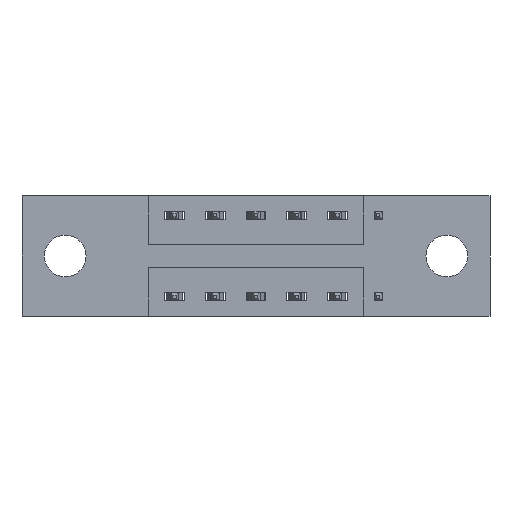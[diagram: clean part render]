
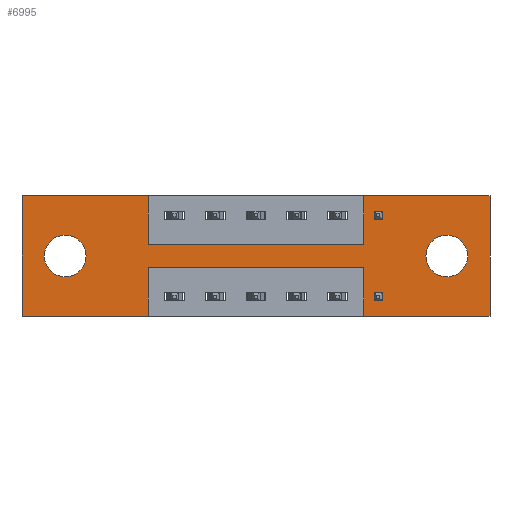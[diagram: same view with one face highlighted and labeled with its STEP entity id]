
A CAD part, front view. The second image highlights one B-rep face of the part: STEP entity #6995.
In plain terms, the highlighted planar face has unit normal (0, -1, 0).
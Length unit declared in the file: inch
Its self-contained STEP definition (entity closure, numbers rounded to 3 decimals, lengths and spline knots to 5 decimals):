
#26 = VERTEX_POINT ( 'NONE', #4920 ) ;
#130 = DIRECTION ( 'NONE',  ( 0., 0., -1. ) ) ;
#154 = CIRCLE ( 'NONE', #3363, 0.064 ) ;
#184 = AXIS2_PLACEMENT_3D ( 'NONE', #5138, #247, #5956 ) ;
#207 = ORIENTED_EDGE ( 'NONE', *, *, #250, .F. ) ;
#247 = DIRECTION ( 'NONE',  ( 0., -1., 0. ) ) ;
#250 = EDGE_CURVE ( 'NONE', #4261, #26, #7551, .T. ) ;
#269 = CARTESIAN_POINT ( 'NONE',  ( 0., 0., 0. ) ) ;
#484 = LINE ( 'NONE', #3034, #7723 ) ;
#500 = VERTEX_POINT ( 'NONE', #683 ) ;
#508 = EDGE_CURVE ( 'NONE', #796, #6614, #5262, .T. ) ;
#578 = AXIS2_PLACEMENT_3D ( 'NONE', #3106, #1083, #6284 ) ;
#643 = EDGE_CURVE ( 'NONE', #3928, #4161, #154, .T. ) ;
#683 = CARTESIAN_POINT ( 'NONE',  ( 0., 0., 0. ) ) ;
#751 = CARTESIAN_POINT ( 'NONE',  ( 1.3025, 0., -0.185 ) ) ;
#796 = VERTEX_POINT ( 'NONE', #7041 ) ;
#982 = ORIENTED_EDGE ( 'NONE', *, *, #6462, .F. ) ;
#998 = ORIENTED_EDGE ( 'NONE', *, *, #5204, .F. ) ;
#1083 = DIRECTION ( 'NONE',  ( 0., 1., 0. ) ) ;
#1354 = ORIENTED_EDGE ( 'NONE', *, *, #7322, .F. ) ;
#1363 = VERTEX_POINT ( 'NONE', #4975 ) ;
#1397 = DIRECTION ( 'NONE',  ( 0., 0., 1. ) ) ;
#1439 = CARTESIAN_POINT ( 'NONE',  ( 1.0475, 0., -0.15 ) ) ;
#1505 = DIRECTION ( 'NONE',  ( 0., 1., 0. ) ) ;
#1611 = ORIENTED_EDGE ( 'NONE', *, *, #8001, .F. ) ;
#1653 = VECTOR ( 'NONE', #5224, 39.37008 ) ;
#1746 = CARTESIAN_POINT ( 'NONE',  ( 1.435, 0., 0. ) ) ;
#1780 = VECTOR ( 'NONE', #1831, 39.37008 ) ;
#1831 = DIRECTION ( 'NONE',  ( 0., 0., 1. ) ) ;
#1835 = VERTEX_POINT ( 'NONE', #4892 ) ;
#1942 = CARTESIAN_POINT ( 'NONE',  ( 1.3025, 0., -0.249 ) ) ;
#2013 = LINE ( 'NONE', #3412, #4089 ) ;
#2039 = VECTOR ( 'NONE', #6839, 39.37008 ) ;
#2126 = LINE ( 'NONE', #2220, #7481 ) ;
#2173 = FACE_BOUND ( 'NONE', #6043, .T. ) ;
#2220 = CARTESIAN_POINT ( 'NONE',  ( 0., 0., -0.37 ) ) ;
#2291 = AXIS2_PLACEMENT_3D ( 'NONE', #4592, #7200, #1397 ) ;
#2400 = LINE ( 'NONE', #1746, #3653 ) ;
#2401 = DIRECTION ( 'NONE',  ( 1., 0., 0. ) ) ;
#2428 = CARTESIAN_POINT ( 'NONE',  ( 0., 0., 0. ) ) ;
#2572 = FACE_BOUND ( 'NONE', #6001, .T. ) ;
#2657 = CARTESIAN_POINT ( 'NONE',  ( 0.3875, 0., 0. ) ) ;
#2852 = DIRECTION ( 'NONE',  ( -1., 0., 0. ) ) ;
#3034 = CARTESIAN_POINT ( 'NONE',  ( 0.3875, 0., -0.37 ) ) ;
#3106 = CARTESIAN_POINT ( 'NONE',  ( 1.3025, 0., -0.185 ) ) ;
#3128 = ORIENTED_EDGE ( 'NONE', *, *, #6945, .F. ) ;
#3243 = EDGE_CURVE ( 'NONE', #6526, #500, #4103, .T. ) ;
#3318 = DIRECTION ( 'NONE',  ( 0., 1., 0. ) ) ;
#3351 = CARTESIAN_POINT ( 'NONE',  ( 0., 0., -0.37 ) ) ;
#3363 = AXIS2_PLACEMENT_3D ( 'NONE', #751, #3318, #130 ) ;
#3412 = CARTESIAN_POINT ( 'NONE',  ( 1.0475, 0., 0. ) ) ;
#3513 = EDGE_CURVE ( 'NONE', #5589, #1835, #5883, .T. ) ;
#3555 = CARTESIAN_POINT ( 'NONE',  ( 1.0475, 0., 0. ) ) ;
#3630 = LINE ( 'NONE', #4946, #5316 ) ;
#3653 = VECTOR ( 'NONE', #4329, 39.37008 ) ;
#3655 = ORIENTED_EDGE ( 'NONE', *, *, #508, .T. ) ;
#3745 = LINE ( 'NONE', #4406, #5836 ) ;
#3862 = ORIENTED_EDGE ( 'NONE', *, *, #6370, .F. ) ;
#3868 = LINE ( 'NONE', #6358, #1780 ) ;
#3928 = VERTEX_POINT ( 'NONE', #6560 ) ;
#4005 = DIRECTION ( 'NONE',  ( -1., 0., 0. ) ) ;
#4089 = VECTOR ( 'NONE', #4628, 39.37008 ) ;
#4103 = LINE ( 'NONE', #269, #5554 ) ;
#4123 = ORIENTED_EDGE ( 'NONE', *, *, #5888, .F. ) ;
#4161 = VERTEX_POINT ( 'NONE', #1942 ) ;
#4261 = VERTEX_POINT ( 'NONE', #3555 ) ;
#4328 = VECTOR ( 'NONE', #4005, 39.37008 ) ;
#4329 = DIRECTION ( 'NONE',  ( 0., 0., -1. ) ) ;
#4406 = CARTESIAN_POINT ( 'NONE',  ( 0., 0., 0. ) ) ;
#4583 = CARTESIAN_POINT ( 'NONE',  ( 0.3875, 0., -0.22 ) ) ;
#4592 = CARTESIAN_POINT ( 'NONE',  ( 0.1325, 0., -0.185 ) ) ;
#4628 = DIRECTION ( 'NONE',  ( 0., 0., 1. ) ) ;
#4744 = CARTESIAN_POINT ( 'NONE',  ( 0.3875, 0., -0.37 ) ) ;
#4803 = DIRECTION ( 'NONE',  ( 0., 0., 1. ) ) ;
#4891 = CARTESIAN_POINT ( 'NONE',  ( 0.3875, 0., -0.15 ) ) ;
#4892 = CARTESIAN_POINT ( 'NONE',  ( 0.3875, 0., -0.15 ) ) ;
#4894 = AXIS2_PLACEMENT_3D ( 'NONE', #7319, #1505, #6663 ) ;
#4920 = CARTESIAN_POINT ( 'NONE',  ( 1.435, 0., 0. ) ) ;
#4946 = CARTESIAN_POINT ( 'NONE',  ( 0., 0., -0.37 ) ) ;
#4975 = CARTESIAN_POINT ( 'NONE',  ( 1.0475, 0., -0.37 ) ) ;
#5138 = CARTESIAN_POINT ( 'NONE',  ( 0., 0., -0.37 ) ) ;
#5180 = EDGE_CURVE ( 'NONE', #4161, #3928, #6217, .T. ) ;
#5204 = EDGE_CURVE ( 'NONE', #26, #7951, #2400, .T. ) ;
#5205 = ORIENTED_EDGE ( 'NONE', *, *, #643, .T. ) ;
#5224 = DIRECTION ( 'NONE',  ( 0., 0., -1. ) ) ;
#5260 = ORIENTED_EDGE ( 'NONE', *, *, #5180, .T. ) ;
#5262 = CIRCLE ( 'NONE', #2291, 0.064 ) ;
#5316 = VECTOR ( 'NONE', #7529, 39.37008 ) ;
#5353 = PLANE ( 'NONE',  #184 ) ;
#5452 = CARTESIAN_POINT ( 'NONE',  ( 1.0475, 0., -0.22 ) ) ;
#5457 = ORIENTED_EDGE ( 'NONE', *, *, #8246, .F. ) ;
#5554 = VECTOR ( 'NONE', #4803, 39.37008 ) ;
#5589 = VERTEX_POINT ( 'NONE', #8318 ) ;
#5612 = DIRECTION ( 'NONE',  ( 0., 0., -1. ) ) ;
#5786 = FACE_OUTER_BOUND ( 'NONE', #6097, .T. ) ;
#5836 = VECTOR ( 'NONE', #2401, 39.37008 ) ;
#5843 = LINE ( 'NONE', #4583, #4328 ) ;
#5883 = LINE ( 'NONE', #2657, #1653 ) ;
#5888 = EDGE_CURVE ( 'NONE', #7228, #6421, #5843, .T. ) ;
#5956 = DIRECTION ( 'NONE',  ( 0., 0., -1. ) ) ;
#6001 = EDGE_LOOP ( 'NONE', ( #5205, #5260 ) ) ;
#6027 = CARTESIAN_POINT ( 'NONE',  ( 1.435, 0., -0.37 ) ) ;
#6043 = EDGE_LOOP ( 'NONE', ( #3655, #6936 ) ) ;
#6097 = EDGE_LOOP ( 'NONE', ( #1354, #4123, #5457, #1611, #998, #207, #3862, #982, #6660, #3128, #7566, #6899 ) ) ;
#6112 = VERTEX_POINT ( 'NONE', #4744 ) ;
#6217 = CIRCLE ( 'NONE', #578, 0.064 ) ;
#6284 = DIRECTION ( 'NONE',  ( 0., 0., -1. ) ) ;
#6349 = DIRECTION ( 'NONE',  ( 1., 0., 0. ) ) ;
#6358 = CARTESIAN_POINT ( 'NONE',  ( 1.0475, 0., -0.37 ) ) ;
#6370 = EDGE_CURVE ( 'NONE', #6994, #4261, #2013, .T. ) ;
#6421 = VERTEX_POINT ( 'NONE', #7359 ) ;
#6462 = EDGE_CURVE ( 'NONE', #1835, #6994, #8122, .T. ) ;
#6526 = VERTEX_POINT ( 'NONE', #3351 ) ;
#6560 = CARTESIAN_POINT ( 'NONE',  ( 1.3025, 0., -0.121 ) ) ;
#6614 = VERTEX_POINT ( 'NONE', #7630 ) ;
#6660 = ORIENTED_EDGE ( 'NONE', *, *, #3513, .F. ) ;
#6663 = DIRECTION ( 'NONE',  ( 0., 0., 1. ) ) ;
#6726 = EDGE_CURVE ( 'NONE', #6112, #6526, #2126, .T. ) ;
#6839 = DIRECTION ( 'NONE',  ( 1., 0., 0. ) ) ;
#6899 = ORIENTED_EDGE ( 'NONE', *, *, #6726, .F. ) ;
#6936 = ORIENTED_EDGE ( 'NONE', *, *, #7735, .T. ) ;
#6945 = EDGE_CURVE ( 'NONE', #500, #5589, #3745, .T. ) ;
#6994 = VERTEX_POINT ( 'NONE', #1439 ) ;
#6995 = ADVANCED_FACE ( 'NONE', ( #2572, #2173, #5786 ), #5353, .T. ) ;
#7041 = CARTESIAN_POINT ( 'NONE',  ( 0.1325, 0., -0.121 ) ) ;
#7157 = VECTOR ( 'NONE', #6349, 39.37008 ) ;
#7200 = DIRECTION ( 'NONE',  ( 0., 1., 0. ) ) ;
#7228 = VERTEX_POINT ( 'NONE', #5452 ) ;
#7319 = CARTESIAN_POINT ( 'NONE',  ( 0.1325, 0., -0.185 ) ) ;
#7322 = EDGE_CURVE ( 'NONE', #6421, #6112, #484, .T. ) ;
#7359 = CARTESIAN_POINT ( 'NONE',  ( 0.3875, 0., -0.22 ) ) ;
#7481 = VECTOR ( 'NONE', #2852, 39.37008 ) ;
#7529 = DIRECTION ( 'NONE',  ( -1., 0., 0. ) ) ;
#7551 = LINE ( 'NONE', #2428, #7157 ) ;
#7566 = ORIENTED_EDGE ( 'NONE', *, *, #3243, .F. ) ;
#7630 = CARTESIAN_POINT ( 'NONE',  ( 0.1325, 0., -0.249 ) ) ;
#7723 = VECTOR ( 'NONE', #5612, 39.37008 ) ;
#7729 = CIRCLE ( 'NONE', #4894, 0.064 ) ;
#7735 = EDGE_CURVE ( 'NONE', #6614, #796, #7729, .T. ) ;
#7951 = VERTEX_POINT ( 'NONE', #6027 ) ;
#8001 = EDGE_CURVE ( 'NONE', #7951, #1363, #3630, .T. ) ;
#8122 = LINE ( 'NONE', #4891, #2039 ) ;
#8246 = EDGE_CURVE ( 'NONE', #1363, #7228, #3868, .T. ) ;
#8318 = CARTESIAN_POINT ( 'NONE',  ( 0.3875, 0., 0. ) ) ;
